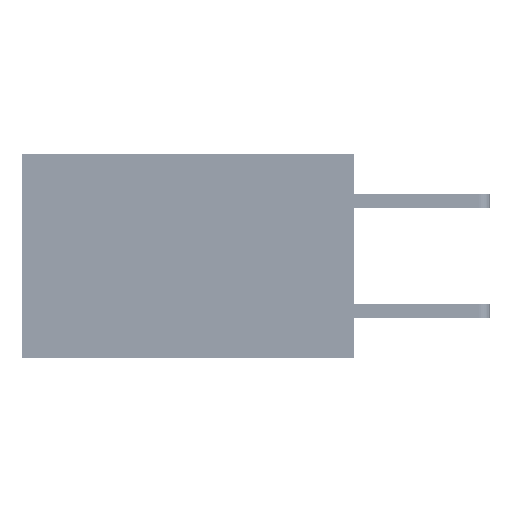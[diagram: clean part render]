
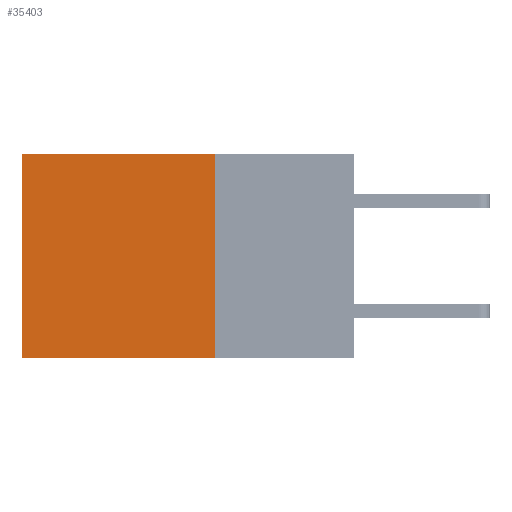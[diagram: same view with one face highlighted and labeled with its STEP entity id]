
A CAD part, left-side view. The second image highlights one B-rep face of the part: STEP entity #35403.
In plain terms, the highlighted planar face has unit normal (-1, 0, 0).
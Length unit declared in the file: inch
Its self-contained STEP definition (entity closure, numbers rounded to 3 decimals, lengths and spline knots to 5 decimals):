
#843 = DIRECTION ( 'NONE',  ( 0., 0., -1. ) ) ;
#3921 = VERTEX_POINT ( 'NONE', #15844 ) ;
#4383 = ORIENTED_EDGE ( 'NONE', *, *, #33837, .F. ) ;
#5058 = EDGE_CURVE ( 'NONE', #43255, #21302, #35349, .T. ) ;
#5720 = ORIENTED_EDGE ( 'NONE', *, *, #6585, .T. ) ;
#6585 = EDGE_CURVE ( 'NONE', #43255, #3921, #26315, .T. ) ;
#7259 = CARTESIAN_POINT ( 'NONE',  ( 0.2875, 0.25, 0. ) ) ;
#9325 = AXIS2_PLACEMENT_3D ( 'NONE', #19578, #37210, #16570 ) ;
#14556 = CARTESIAN_POINT ( 'NONE',  ( 0.2875, 0.6, -0.37 ) ) ;
#15407 = EDGE_CURVE ( 'NONE', #3921, #26453, #32974, .T. ) ;
#15627 = CARTESIAN_POINT ( 'NONE',  ( 0.2875, 0.25, -0.37 ) ) ;
#15844 = CARTESIAN_POINT ( 'NONE',  ( 0.2875, 0.6, 0. ) ) ;
#16094 = CARTESIAN_POINT ( 'NONE',  ( 0.2875, 0.25, 0. ) ) ;
#16570 = DIRECTION ( 'NONE',  ( 0., 0., -1. ) ) ;
#16855 = CARTESIAN_POINT ( 'NONE',  ( 0.2875, 0.6, 0. ) ) ;
#17524 = VECTOR ( 'NONE', #39774, 39.37008 ) ;
#19578 = CARTESIAN_POINT ( 'NONE',  ( 0.2875, 0.25, 0. ) ) ;
#21302 = VERTEX_POINT ( 'NONE', #23374 ) ;
#21417 = ORIENTED_EDGE ( 'NONE', *, *, #5058, .F. ) ;
#22714 = VECTOR ( 'NONE', #37506, 39.37008 ) ;
#23374 = CARTESIAN_POINT ( 'NONE',  ( 0.2875, 0.25, -0.37 ) ) ;
#26179 = VECTOR ( 'NONE', #843, 39.37008 ) ;
#26238 = EDGE_LOOP ( 'NONE', ( #26698, #4383, #21417, #5720 ) ) ;
#26315 = LINE ( 'NONE', #7259, #34407 ) ;
#26453 = VERTEX_POINT ( 'NONE', #14556 ) ;
#26698 = ORIENTED_EDGE ( 'NONE', *, *, #15407, .T. ) ;
#28146 = FACE_OUTER_BOUND ( 'NONE', #26238, .T. ) ;
#32974 = LINE ( 'NONE', #16855, #22714 ) ;
#33730 = PLANE ( 'NONE',  #9325 ) ;
#33837 = EDGE_CURVE ( 'NONE', #21302, #26453, #43930, .T. ) ;
#34407 = VECTOR ( 'NONE', #41600, 39.37008 ) ;
#35197 = CARTESIAN_POINT ( 'NONE',  ( 0.2875, 0.25, 0. ) ) ;
#35349 = LINE ( 'NONE', #35197, #26179 ) ;
#35403 = ADVANCED_FACE ( 'NONE', ( #28146 ), #33730, .F. ) ;
#37210 = DIRECTION ( 'NONE',  ( 1., 0., 0. ) ) ;
#37506 = DIRECTION ( 'NONE',  ( 0., 0., -1. ) ) ;
#39774 = DIRECTION ( 'NONE',  ( 0., 1., 0. ) ) ;
#41600 = DIRECTION ( 'NONE',  ( 0., 1., 0. ) ) ;
#43255 = VERTEX_POINT ( 'NONE', #16094 ) ;
#43930 = LINE ( 'NONE', #15627, #17524 ) ;
